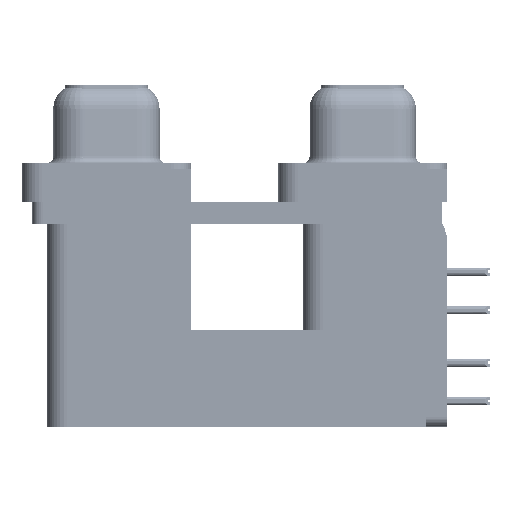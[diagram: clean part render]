
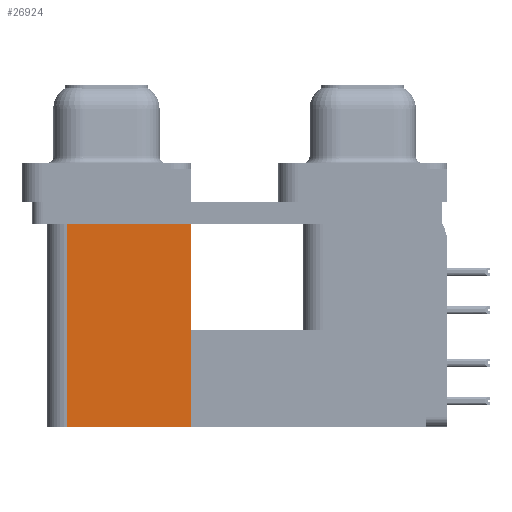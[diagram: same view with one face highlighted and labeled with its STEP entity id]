
A CAD part, left-side view. The second image highlights one B-rep face of the part: STEP entity #26924.
In plain terms, the highlighted planar face has unit normal (-1, 0, 0).
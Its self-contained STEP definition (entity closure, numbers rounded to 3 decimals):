
#4045 = CARTESIAN_POINT ( 'NONE',  ( 3.79, 21.975, -19.2 ) ) ;
#4054 = LINE ( 'NONE', #54304, #13500 ) ;
#4393 = VERTEX_POINT ( 'NONE', #57460 ) ;
#7285 = DIRECTION ( 'NONE',  ( 0., 1., 0. ) ) ;
#9466 = FACE_OUTER_BOUND ( 'NONE', #19790, .T. ) ;
#10138 = CARTESIAN_POINT ( 'NONE',  ( 3.79, 21.975, -19.2 ) ) ;
#10713 = CARTESIAN_POINT ( 'NONE',  ( 3.79, 21.975, -2.5 ) ) ;
#12896 = VERTEX_POINT ( 'NONE', #10713 ) ;
#13500 = VECTOR ( 'NONE', #26271, 1000. ) ;
#13843 = VERTEX_POINT ( 'NONE', #46445 ) ;
#15962 = LINE ( 'NONE', #10138, #47613 ) ;
#19790 = EDGE_LOOP ( 'NONE', ( #48750, #30782, #48036, #59696 ) ) ;
#22431 = VECTOR ( 'NONE', #56743, 1000. ) ;
#26271 = DIRECTION ( 'NONE',  ( 0., 0., 1. ) ) ;
#26924 = ADVANCED_FACE ( 'NONE', ( #9466 ), #70997, .F. ) ;
#30782 = ORIENTED_EDGE ( 'NONE', *, *, #49715, .F. ) ;
#31689 = CARTESIAN_POINT ( 'NONE',  ( 3.79, 12.775, -19.2 ) ) ;
#32214 = EDGE_CURVE ( 'NONE', #4393, #12896, #40049, .T. ) ;
#32532 = AXIS2_PLACEMENT_3D ( 'NONE', #31689, #47341, #53912 ) ;
#33568 = VECTOR ( 'NONE', #7285, 1000. ) ;
#35669 = CARTESIAN_POINT ( 'NONE',  ( 3.79, 12.775, -2.5 ) ) ;
#40049 = LINE ( 'NONE', #35669, #33568 ) ;
#43633 = VERTEX_POINT ( 'NONE', #4045 ) ;
#46445 = CARTESIAN_POINT ( 'NONE',  ( 3.79, 12.775, -19.2 ) ) ;
#47341 = DIRECTION ( 'NONE',  ( 1., 0., 0. ) ) ;
#47613 = VECTOR ( 'NONE', #55309, 1000. ) ;
#48036 = ORIENTED_EDGE ( 'NONE', *, *, #71335, .F. ) ;
#48750 = ORIENTED_EDGE ( 'NONE', *, *, #32214, .T. ) ;
#49715 = EDGE_CURVE ( 'NONE', #43633, #12896, #15962, .T. ) ;
#52372 = LINE ( 'NONE', #63319, #22431 ) ;
#53912 = DIRECTION ( 'NONE',  ( 0., 0., -1. ) ) ;
#54304 = CARTESIAN_POINT ( 'NONE',  ( 3.79, 12.775, -19.2 ) ) ;
#55309 = DIRECTION ( 'NONE',  ( 0., 0., 1. ) ) ;
#56743 = DIRECTION ( 'NONE',  ( 0., 1., 0. ) ) ;
#57460 = CARTESIAN_POINT ( 'NONE',  ( 3.79, 12.775, -2.5 ) ) ;
#59492 = EDGE_CURVE ( 'NONE', #13843, #4393, #4054, .T. ) ;
#59696 = ORIENTED_EDGE ( 'NONE', *, *, #59492, .T. ) ;
#63319 = CARTESIAN_POINT ( 'NONE',  ( 3.79, 12.775, -19.2 ) ) ;
#70997 = PLANE ( 'NONE',  #32532 ) ;
#71335 = EDGE_CURVE ( 'NONE', #13843, #43633, #52372, .T. ) ;
